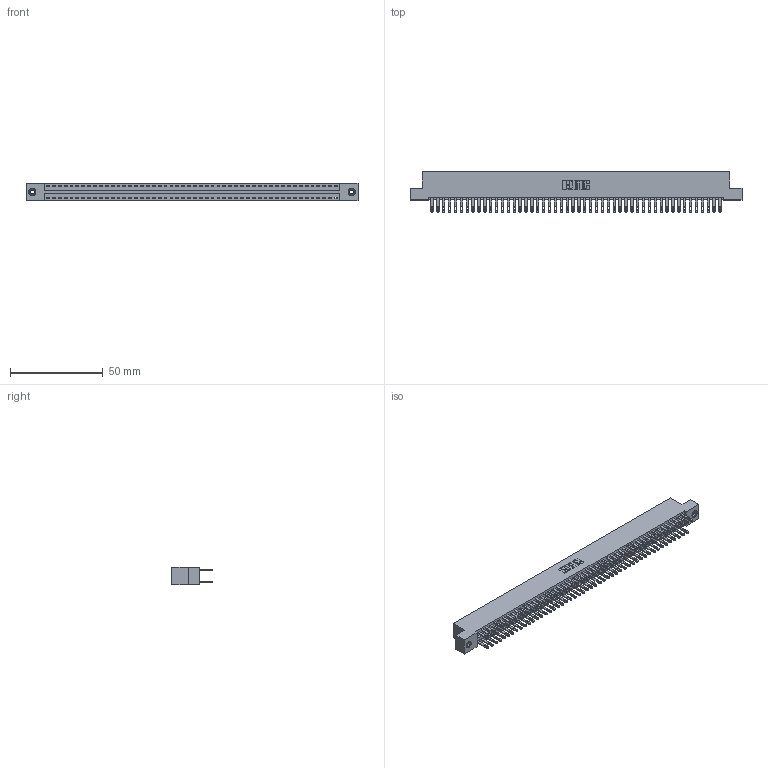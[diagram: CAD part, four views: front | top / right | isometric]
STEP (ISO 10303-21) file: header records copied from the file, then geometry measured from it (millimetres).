
FILE_DESCRIPTION (( 'STEP AP203' ), '1' );
FILE_NAME ('896-100-500-208.STEP', '2021-07-28T03:44:50', ( '' ), ( '' ), 'SwSTEP 2.0', 'SolidWorks 2020', '' );
FILE_SCHEMA (( 'CONFIG_CONTROL_DESIGN' ));
Length unit declared in the file: inch
Products named in the file (4): 345-250-001_345-250-003-102; 345-292-001_345-293-100; 896-100-500-208; 846 Part_Flush Mounting Lugs - 0.156 Dia-TI
Assembly tree (102 placements, depth 2):
  896-100-500-208
    846 Part_Flush Mounting Lugs - 0.156 Dia-TI
    345-292-001_345-293-100  x99
    345-250-001_345-250-003-102  x2
Bounding box: 179.32 x 21.84 x 9.4 mm (x, y, z)
Volume: 17835.5 mm3; surface area: 25646.1 mm2
Topology: 102 solids, 102 shells, 4940 faces, 15039 edges, 10018 vertices
Faces by surface type: plane 2984, cylinder 1940, cone 12, torus 4
Entity records: 32638 total; most frequent: CARTESIAN_POINT 5354, ORIENTED_EDGE 5282, DIRECTION 4797, EDGE_CURVE 2641, LINE 2285, VECTOR 2285, VERTEX_POINT 1756, AXIS2_PLACEMENT_3D 1256
